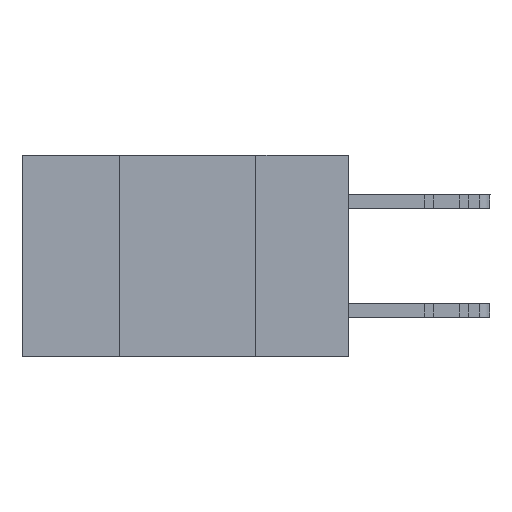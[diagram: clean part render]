
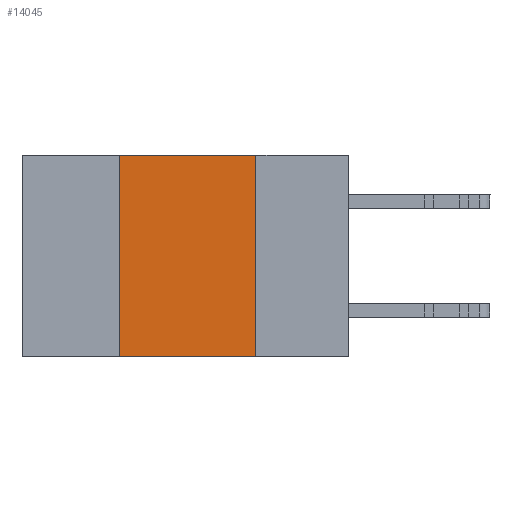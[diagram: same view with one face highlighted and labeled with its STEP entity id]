
A CAD part, left-side view. The second image highlights one B-rep face of the part: STEP entity #14045.
In plain terms, the highlighted planar face has unit normal (-1, 0, 0).
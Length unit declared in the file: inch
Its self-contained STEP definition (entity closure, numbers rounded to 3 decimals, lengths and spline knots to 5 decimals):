
#1526 = DIRECTION ( 'NONE',  ( 0., 0., -1. ) ) ;
#1772 = DIRECTION ( 'NONE',  ( 0., 0., 1. ) ) ;
#1938 = DIRECTION ( 'NONE',  ( 0., -1., 0. ) ) ;
#2107 = VERTEX_POINT ( 'NONE', #3153 ) ;
#3153 = CARTESIAN_POINT ( 'NONE',  ( 0., 0.42, 0. ) ) ;
#3943 = CARTESIAN_POINT ( 'NONE',  ( 0., 0.17, 0. ) ) ;
#4506 = VECTOR ( 'NONE', #1772, 39.37008 ) ;
#4711 = EDGE_CURVE ( 'NONE', #21964, #2107, #9844, .T. ) ;
#4910 = LINE ( 'NONE', #31875, #10430 ) ;
#6385 = ORIENTED_EDGE ( 'NONE', *, *, #4711, .F. ) ;
#6870 = EDGE_LOOP ( 'NONE', ( #25024, #7150, #6385, #26144 ) ) ;
#6881 = VERTEX_POINT ( 'NONE', #24151 ) ;
#7127 = VECTOR ( 'NONE', #1938, 39.37008 ) ;
#7144 = PLANE ( 'NONE',  #8723 ) ;
#7150 = ORIENTED_EDGE ( 'NONE', *, *, #19200, .F. ) ;
#8723 = AXIS2_PLACEMENT_3D ( 'NONE', #28799, #31373, #31848 ) ;
#9376 = CARTESIAN_POINT ( 'NONE',  ( 0., 0.6, -0.37 ) ) ;
#9844 = LINE ( 'NONE', #19677, #4506 ) ;
#10402 = CARTESIAN_POINT ( 'NONE',  ( 0., 0.42, -0.37 ) ) ;
#10430 = VECTOR ( 'NONE', #12508, 39.37008 ) ;
#12508 = DIRECTION ( 'NONE',  ( 0., -1., 0. ) ) ;
#14045 = ADVANCED_FACE ( 'NONE', ( #18919 ), #7144, .F. ) ;
#14218 = LINE ( 'NONE', #9376, #7127 ) ;
#15888 = CARTESIAN_POINT ( 'NONE',  ( 0., 0.17, 0. ) ) ;
#18125 = VECTOR ( 'NONE', #1526, 39.37008 ) ;
#18627 = LINE ( 'NONE', #3943, #18125 ) ;
#18919 = FACE_OUTER_BOUND ( 'NONE', #6870, .T. ) ;
#19024 = EDGE_CURVE ( 'NONE', #22021, #6881, #18627, .T. ) ;
#19200 = EDGE_CURVE ( 'NONE', #2107, #22021, #4910, .T. ) ;
#19677 = CARTESIAN_POINT ( 'NONE',  ( 0., 0.42, 0. ) ) ;
#21964 = VERTEX_POINT ( 'NONE', #10402 ) ;
#22021 = VERTEX_POINT ( 'NONE', #15888 ) ;
#24151 = CARTESIAN_POINT ( 'NONE',  ( 0., 0.17, -0.37 ) ) ;
#25024 = ORIENTED_EDGE ( 'NONE', *, *, #19024, .F. ) ;
#26144 = ORIENTED_EDGE ( 'NONE', *, *, #29363, .T. ) ;
#28799 = CARTESIAN_POINT ( 'NONE',  ( 0., 0.6, 0. ) ) ;
#29363 = EDGE_CURVE ( 'NONE', #21964, #6881, #14218, .T. ) ;
#31373 = DIRECTION ( 'NONE',  ( 1., 0., 0. ) ) ;
#31848 = DIRECTION ( 'NONE',  ( 0., 0., -1. ) ) ;
#31875 = CARTESIAN_POINT ( 'NONE',  ( 0., 0.6, 0. ) ) ;
